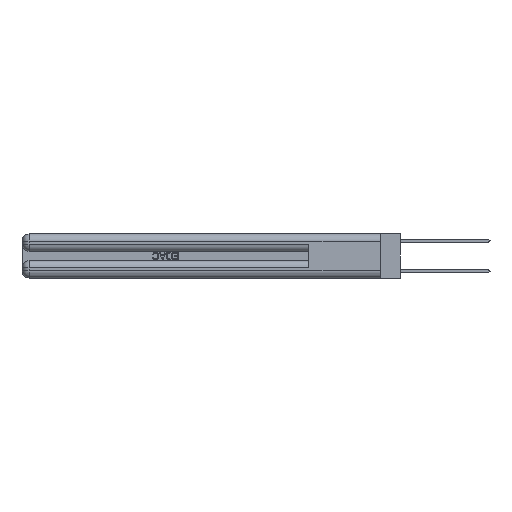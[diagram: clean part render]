
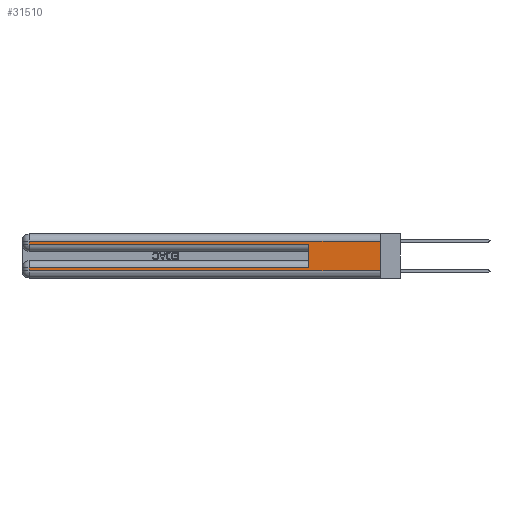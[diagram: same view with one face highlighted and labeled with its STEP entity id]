
A CAD part, left-side view. The second image highlights one B-rep face of the part: STEP entity #31510.
In plain terms, the highlighted planar face has unit normal (-1, 0, 0).
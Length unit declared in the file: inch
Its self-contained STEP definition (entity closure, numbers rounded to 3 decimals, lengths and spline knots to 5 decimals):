
#147 = AXIS2_PLACEMENT_3D ( 'NONE', #4199, #14754, #25337 ) ;
#498 = VECTOR ( 'NONE', #26043, 39.37008 ) ;
#1247 = VECTOR ( 'NONE', #30203, 39.37008 ) ;
#3237 = LINE ( 'NONE', #26642, #12408 ) ;
#3370 = EDGE_LOOP ( 'NONE', ( #12352, #5282, #29119, #14985, #25237, #12714, #10098, #9388 ) ) ;
#3755 = VERTEX_POINT ( 'NONE', #12180 ) ;
#4199 = CARTESIAN_POINT ( 'NONE',  ( 0., 0., 0.37 ) ) ;
#4384 = CARTESIAN_POINT ( 'NONE',  ( 0., 2.94, 0.37 ) ) ;
#4478 = CARTESIAN_POINT ( 'NONE',  ( 0., 2.94, 0.285 ) ) ;
#4780 = VERTEX_POINT ( 'NONE', #4478 ) ;
#4843 = EDGE_CURVE ( 'NONE', #27967, #3755, #17630, .T. ) ;
#4949 = EDGE_CURVE ( 'NONE', #24856, #29082, #3237, .T. ) ;
#5257 = LINE ( 'NONE', #18937, #9412 ) ;
#5282 = ORIENTED_EDGE ( 'NONE', *, *, #4843, .T. ) ;
#5739 = VECTOR ( 'NONE', #33751, 39.37008 ) ;
#5834 = DIRECTION ( 'NONE',  ( 0., 0., 1. ) ) ;
#6580 = LINE ( 'NONE', #9699, #34168 ) ;
#6789 = PLANE ( 'NONE',  #147 ) ;
#9388 = ORIENTED_EDGE ( 'NONE', *, *, #26162, .T. ) ;
#9412 = VECTOR ( 'NONE', #23795, 39.37008 ) ;
#9482 = EDGE_CURVE ( 'NONE', #24856, #20915, #23899, .T. ) ;
#9699 = CARTESIAN_POINT ( 'NONE',  ( 0., 0., 0.285 ) ) ;
#10098 = ORIENTED_EDGE ( 'NONE', *, *, #25131, .T. ) ;
#11583 = EDGE_CURVE ( 'NONE', #4780, #29082, #6580, .T. ) ;
#12180 = CARTESIAN_POINT ( 'NONE',  ( 0., 2.94, 0.31 ) ) ;
#12352 = ORIENTED_EDGE ( 'NONE', *, *, #25500, .F. ) ;
#12408 = VECTOR ( 'NONE', #5834, 39.37008 ) ;
#12714 = ORIENTED_EDGE ( 'NONE', *, *, #9482, .T. ) ;
#12730 = CARTESIAN_POINT ( 'NONE',  ( 0., 0.6, 0.285 ) ) ;
#13877 = LINE ( 'NONE', #27751, #24324 ) ;
#14754 = DIRECTION ( 'NONE',  ( 1., 0., 0. ) ) ;
#14886 = DIRECTION ( 'NONE',  ( 0., -1., 0. ) ) ;
#14985 = ORIENTED_EDGE ( 'NONE', *, *, #11583, .T. ) ;
#15373 = CARTESIAN_POINT ( 'NONE',  ( 0., 0., 0.31 ) ) ;
#16651 = DIRECTION ( 'NONE',  ( 0., 0., -1. ) ) ;
#17630 = LINE ( 'NONE', #15373, #5739 ) ;
#18937 = CARTESIAN_POINT ( 'NONE',  ( 0., 0., 0.06 ) ) ;
#19791 = VECTOR ( 'NONE', #21292, 39.37008 ) ;
#20780 = CARTESIAN_POINT ( 'NONE',  ( 0., 0., 0.085 ) ) ;
#20915 = VERTEX_POINT ( 'NONE', #30401 ) ;
#21292 = DIRECTION ( 'NONE',  ( 0., 1., 0. ) ) ;
#21302 = VERTEX_POINT ( 'NONE', #21879 ) ;
#21879 = CARTESIAN_POINT ( 'NONE',  ( 0., 2.94, 0.06 ) ) ;
#23795 = DIRECTION ( 'NONE',  ( 0., -1., 0. ) ) ;
#23899 = LINE ( 'NONE', #20780, #19791 ) ;
#24279 = VERTEX_POINT ( 'NONE', #33623 ) ;
#24324 = VECTOR ( 'NONE', #16651, 39.37008 ) ;
#24856 = VERTEX_POINT ( 'NONE', #26252 ) ;
#25131 = EDGE_CURVE ( 'NONE', #20915, #21302, #25356, .T. ) ;
#25237 = ORIENTED_EDGE ( 'NONE', *, *, #4949, .F. ) ;
#25337 = DIRECTION ( 'NONE',  ( 0., 0., -1. ) ) ;
#25356 = LINE ( 'NONE', #31242, #498 ) ;
#25500 = EDGE_CURVE ( 'NONE', #27967, #24279, #13877, .T. ) ;
#26043 = DIRECTION ( 'NONE',  ( 0., 0., -1. ) ) ;
#26162 = EDGE_CURVE ( 'NONE', #21302, #24279, #5257, .T. ) ;
#26252 = CARTESIAN_POINT ( 'NONE',  ( 0., 0.6, 0.085 ) ) ;
#26642 = CARTESIAN_POINT ( 'NONE',  ( 0., 0.6, 0.145 ) ) ;
#27751 = CARTESIAN_POINT ( 'NONE',  ( 0., 0., 0.37 ) ) ;
#27939 = FACE_OUTER_BOUND ( 'NONE', #3370, .T. ) ;
#27967 = VERTEX_POINT ( 'NONE', #33864 ) ;
#29082 = VERTEX_POINT ( 'NONE', #12730 ) ;
#29119 = ORIENTED_EDGE ( 'NONE', *, *, #29403, .T. ) ;
#29403 = EDGE_CURVE ( 'NONE', #3755, #4780, #33150, .T. ) ;
#30203 = DIRECTION ( 'NONE',  ( 0., 0., -1. ) ) ;
#30401 = CARTESIAN_POINT ( 'NONE',  ( 0., 2.94, 0.085 ) ) ;
#31242 = CARTESIAN_POINT ( 'NONE',  ( 0., 2.94, 0.37 ) ) ;
#31510 = ADVANCED_FACE ( 'NONE', ( #27939 ), #6789, .F. ) ;
#33150 = LINE ( 'NONE', #4384, #1247 ) ;
#33623 = CARTESIAN_POINT ( 'NONE',  ( 0., 0., 0.06 ) ) ;
#33751 = DIRECTION ( 'NONE',  ( 0., 1., 0. ) ) ;
#33864 = CARTESIAN_POINT ( 'NONE',  ( 0., 0., 0.31 ) ) ;
#34168 = VECTOR ( 'NONE', #14886, 39.37008 ) ;
